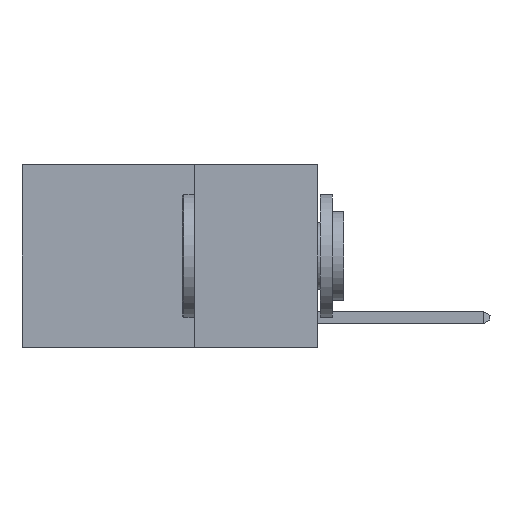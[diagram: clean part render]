
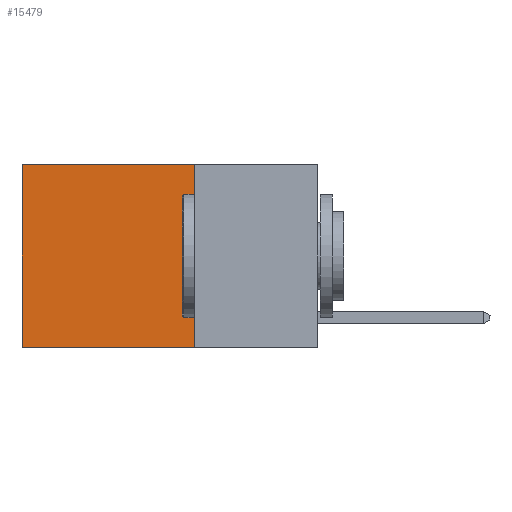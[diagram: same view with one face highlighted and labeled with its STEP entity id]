
A CAD part, left-side view. The second image highlights one B-rep face of the part: STEP entity #15479.
In plain terms, the highlighted planar face has unit normal (-1, 0, 0).
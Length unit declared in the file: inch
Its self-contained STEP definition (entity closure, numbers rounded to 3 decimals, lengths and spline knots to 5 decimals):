
#305 = CARTESIAN_POINT ( 'NONE',  ( 0.2625, 0.25, 0. ) ) ;
#318 = CARTESIAN_POINT ( 'NONE',  ( 0.2625, 0.6, 0. ) ) ;
#406 = ORIENTED_EDGE ( 'NONE', *, *, #4934, .T. ) ;
#465 = AXIS2_PLACEMENT_3D ( 'NONE', #4912, #13179, #6142 ) ;
#869 = VERTEX_POINT ( 'NONE', #318 ) ;
#1591 = ORIENTED_EDGE ( 'NONE', *, *, #12918, .F. ) ;
#2897 = DIRECTION ( 'NONE',  ( 0., 0., -1. ) ) ;
#3092 = LINE ( 'NONE', #7901, #15307 ) ;
#3302 = ORIENTED_EDGE ( 'NONE', *, *, #11174, .F. ) ;
#3420 = LINE ( 'NONE', #305, #12547 ) ;
#3700 = CARTESIAN_POINT ( 'NONE',  ( 0.2625, 0.6, -0.37 ) ) ;
#4912 = CARTESIAN_POINT ( 'NONE',  ( 0.2625, 0.25, 0. ) ) ;
#4934 = EDGE_CURVE ( 'NONE', #6926, #869, #5101, .T. ) ;
#5101 = LINE ( 'NONE', #7049, #13758 ) ;
#6012 = CARTESIAN_POINT ( 'NONE',  ( 0.2625, 0.6, 0. ) ) ;
#6142 = DIRECTION ( 'NONE',  ( 0., 0., -1. ) ) ;
#6926 = VERTEX_POINT ( 'NONE', #15023 ) ;
#7049 = CARTESIAN_POINT ( 'NONE',  ( 0.2625, 0.25, 0. ) ) ;
#7632 = ORIENTED_EDGE ( 'NONE', *, *, #13262, .T. ) ;
#7901 = CARTESIAN_POINT ( 'NONE',  ( 0.2625, 0.25, -0.37 ) ) ;
#8306 = VERTEX_POINT ( 'NONE', #3700 ) ;
#9966 = VERTEX_POINT ( 'NONE', #13286 ) ;
#10272 = EDGE_LOOP ( 'NONE', ( #7632, #3302, #1591, #406 ) ) ;
#11174 = EDGE_CURVE ( 'NONE', #9966, #8306, #3092, .T. ) ;
#12027 = PLANE ( 'NONE',  #465 ) ;
#12034 = VECTOR ( 'NONE', #13068, 39.37008 ) ;
#12547 = VECTOR ( 'NONE', #2897, 39.37008 ) ;
#12872 = DIRECTION ( 'NONE',  ( 0., 1., 0. ) ) ;
#12918 = EDGE_CURVE ( 'NONE', #6926, #9966, #3420, .T. ) ;
#13059 = FACE_OUTER_BOUND ( 'NONE', #10272, .T. ) ;
#13068 = DIRECTION ( 'NONE',  ( 0., 0., -1. ) ) ;
#13179 = DIRECTION ( 'NONE',  ( 1., 0., 0. ) ) ;
#13262 = EDGE_CURVE ( 'NONE', #869, #8306, #15065, .T. ) ;
#13286 = CARTESIAN_POINT ( 'NONE',  ( 0.2625, 0.25, -0.37 ) ) ;
#13716 = DIRECTION ( 'NONE',  ( 0., 1., 0. ) ) ;
#13758 = VECTOR ( 'NONE', #12872, 39.37008 ) ;
#15023 = CARTESIAN_POINT ( 'NONE',  ( 0.2625, 0.25, 0. ) ) ;
#15065 = LINE ( 'NONE', #6012, #12034 ) ;
#15307 = VECTOR ( 'NONE', #13716, 39.37008 ) ;
#15479 = ADVANCED_FACE ( 'NONE', ( #13059 ), #12027, .F. ) ;
